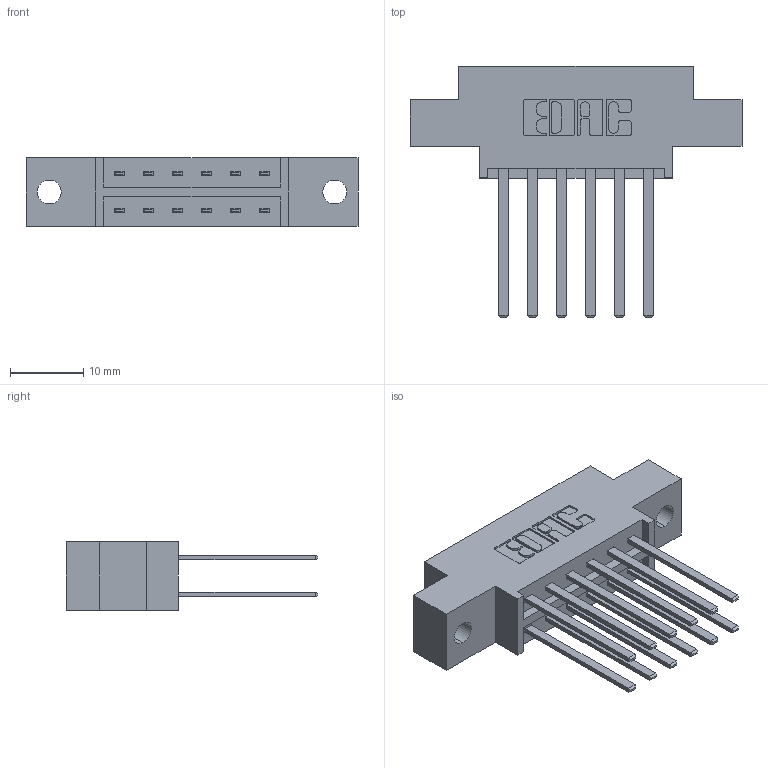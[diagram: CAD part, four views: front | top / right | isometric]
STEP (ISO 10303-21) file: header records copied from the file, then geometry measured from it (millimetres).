
FILE_DESCRIPTION (( 'STEP AP203' ), '1' );
FILE_NAME ('333-012-544-802.STEP', '2018-08-01T00:40:41', ( '' ), ( '' ), 'SwSTEP 2.0', 'SolidWorks 2016', '' );
FILE_SCHEMA (( 'CONFIG_CONTROL_DESIGN' ));
Length unit declared in the file: inch
Products named in the file (3): 333 Part_Offset - .128 Dia; 345-292-001_345-293-144; 333-012-544-802
Assembly tree (13 placements, depth 2):
  333-012-544-802
    333 Part_Offset - .128 Dia
    345-292-001_345-293-144  x12
Bounding box: 45.31 x 34.3 x 9.4 mm (x, y, z)
Volume: 4193.3 mm3; surface area: 5059.9 mm2
Topology: 13 solids, 13 shells, 670 faces, 1967 edges, 1294 vertices
Faces by surface type: plane 458, cylinder 212
Entity records: 8467 total; most frequent: CARTESIAN_POINT 1446, ORIENTED_EDGE 1382, DIRECTION 1295, EDGE_CURVE 691, LINE 567, VECTOR 567, VERTEX_POINT 458, AXIS2_PLACEMENT_3D 364
